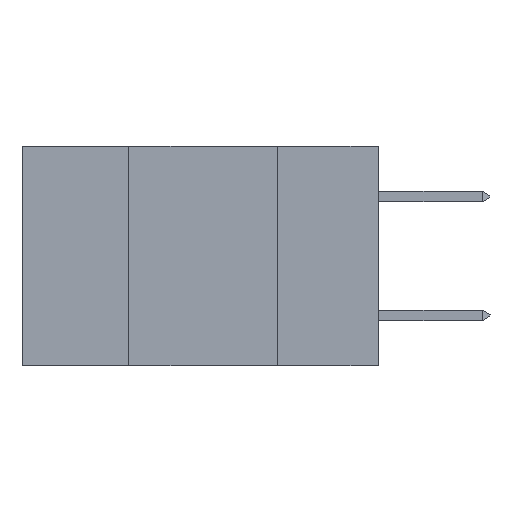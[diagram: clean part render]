
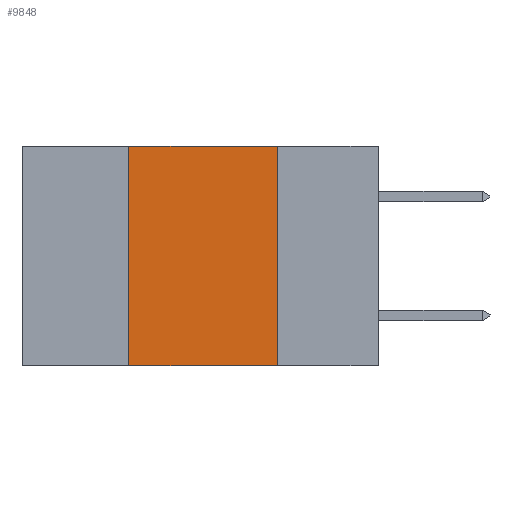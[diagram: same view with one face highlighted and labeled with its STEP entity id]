
A CAD part, left-side view. The second image highlights one B-rep face of the part: STEP entity #9848.
In plain terms, the highlighted planar face has unit normal (-1, 0, 0).
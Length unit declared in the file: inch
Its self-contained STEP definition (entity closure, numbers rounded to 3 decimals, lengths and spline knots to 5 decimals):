
#584 = VECTOR ( 'NONE', #23674, 39.37008 ) ;
#1109 = ORIENTED_EDGE ( 'NONE', *, *, #15880, .F. ) ;
#3208 = VERTEX_POINT ( 'NONE', #6212 ) ;
#3573 = EDGE_CURVE ( 'NONE', #3208, #18652, #20680, .T. ) ;
#3844 = DIRECTION ( 'NONE',  ( 0., 0., -1. ) ) ;
#4778 = ORIENTED_EDGE ( 'NONE', *, *, #14959, .T. ) ;
#5794 = VECTOR ( 'NONE', #7360, 39.37008 ) ;
#6212 = CARTESIAN_POINT ( 'NONE',  ( 0., 0.17, 0. ) ) ;
#7360 = DIRECTION ( 'NONE',  ( 0., -1., 0. ) ) ;
#7478 = DIRECTION ( 'NONE',  ( 0., -1., 0. ) ) ;
#9199 = ORIENTED_EDGE ( 'NONE', *, *, #23203, .F. ) ;
#9272 = VERTEX_POINT ( 'NONE', #11227 ) ;
#9848 = ADVANCED_FACE ( 'NONE', ( #20014 ), #19325, .F. ) ;
#11227 = CARTESIAN_POINT ( 'NONE',  ( 0., 0.42, -0.37 ) ) ;
#11319 = CARTESIAN_POINT ( 'NONE',  ( 0., 0.17, -0.37 ) ) ;
#11393 = CARTESIAN_POINT ( 'NONE',  ( 0., 0.6, 0. ) ) ;
#11808 = CARTESIAN_POINT ( 'NONE',  ( 0., 0.42, 0. ) ) ;
#12667 = AXIS2_PLACEMENT_3D ( 'NONE', #15128, #15211, #3844 ) ;
#13251 = LINE ( 'NONE', #11808, #584 ) ;
#13929 = VECTOR ( 'NONE', #7478, 39.37008 ) ;
#14959 = EDGE_CURVE ( 'NONE', #9272, #18652, #21781, .T. ) ;
#15128 = CARTESIAN_POINT ( 'NONE',  ( 0., 0.6, 0. ) ) ;
#15211 = DIRECTION ( 'NONE',  ( 1., 0., 0. ) ) ;
#15397 = ORIENTED_EDGE ( 'NONE', *, *, #3573, .F. ) ;
#15880 = EDGE_CURVE ( 'NONE', #18882, #3208, #18100, .T. ) ;
#16842 = DIRECTION ( 'NONE',  ( 0., 0., -1. ) ) ;
#18100 = LINE ( 'NONE', #11393, #5794 ) ;
#18128 = EDGE_LOOP ( 'NONE', ( #15397, #1109, #9199, #4778 ) ) ;
#18652 = VERTEX_POINT ( 'NONE', #11319 ) ;
#18882 = VERTEX_POINT ( 'NONE', #20273 ) ;
#18971 = CARTESIAN_POINT ( 'NONE',  ( 0., 0.6, -0.37 ) ) ;
#19325 = PLANE ( 'NONE',  #12667 ) ;
#20014 = FACE_OUTER_BOUND ( 'NONE', #18128, .T. ) ;
#20273 = CARTESIAN_POINT ( 'NONE',  ( 0., 0.42, 0. ) ) ;
#20680 = LINE ( 'NONE', #22680, #21004 ) ;
#21004 = VECTOR ( 'NONE', #16842, 39.37008 ) ;
#21781 = LINE ( 'NONE', #18971, #13929 ) ;
#22680 = CARTESIAN_POINT ( 'NONE',  ( 0., 0.17, 0. ) ) ;
#23203 = EDGE_CURVE ( 'NONE', #9272, #18882, #13251, .T. ) ;
#23674 = DIRECTION ( 'NONE',  ( 0., 0., 1. ) ) ;
